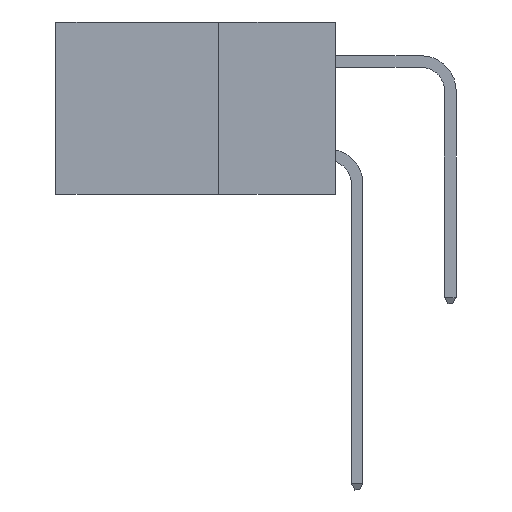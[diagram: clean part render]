
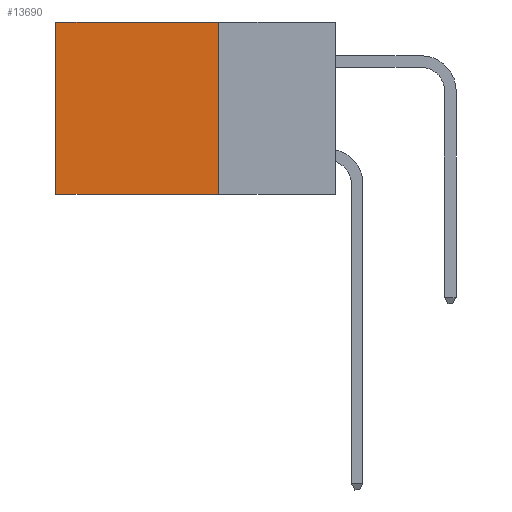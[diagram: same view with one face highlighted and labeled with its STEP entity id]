
A CAD part, left-side view. The second image highlights one B-rep face of the part: STEP entity #13690.
In plain terms, the highlighted planar face has unit normal (-1, 0, 0).
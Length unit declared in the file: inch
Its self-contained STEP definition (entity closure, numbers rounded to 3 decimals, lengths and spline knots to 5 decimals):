
#138 = DIRECTION ( 'NONE',  ( 0., 0., -1. ) ) ;
#770 = LINE ( 'NONE', #13454, #14005 ) ;
#819 = VERTEX_POINT ( 'NONE', #2191 ) ;
#1074 = PLANE ( 'NONE',  #18444 ) ;
#1243 = VECTOR ( 'NONE', #16279, 39.37008 ) ;
#2191 = CARTESIAN_POINT ( 'NONE',  ( 0.2875, 0.25, 0. ) ) ;
#2360 = DIRECTION ( 'NONE',  ( 0., 1., 0. ) ) ;
#2567 = EDGE_CURVE ( 'NONE', #5842, #14217, #11339, .T. ) ;
#2846 = DIRECTION ( 'NONE',  ( 1., 0., 0. ) ) ;
#4188 = EDGE_CURVE ( 'NONE', #8565, #14217, #14970, .T. ) ;
#4939 = ORIENTED_EDGE ( 'NONE', *, *, #13810, .F. ) ;
#5367 = CARTESIAN_POINT ( 'NONE',  ( 0.2875, 0.6, 0. ) ) ;
#5842 = VERTEX_POINT ( 'NONE', #19831 ) ;
#6802 = VECTOR ( 'NONE', #138, 39.37008 ) ;
#8030 = CARTESIAN_POINT ( 'NONE',  ( 0.2875, 0.25, 0. ) ) ;
#8565 = VERTEX_POINT ( 'NONE', #13923 ) ;
#10708 = ORIENTED_EDGE ( 'NONE', *, *, #4188, .F. ) ;
#11164 = CARTESIAN_POINT ( 'NONE',  ( 0.2875, 0.25, -0.37 ) ) ;
#11339 = LINE ( 'NONE', #5367, #6802 ) ;
#12298 = EDGE_CURVE ( 'NONE', #819, #5842, #13822, .T. ) ;
#12642 = EDGE_LOOP ( 'NONE', ( #20370, #10708, #4939, #18631 ) ) ;
#13294 = VECTOR ( 'NONE', #2360, 39.37008 ) ;
#13454 = CARTESIAN_POINT ( 'NONE',  ( 0.2875, 0.25, 0. ) ) ;
#13690 = ADVANCED_FACE ( 'NONE', ( #15603 ), #1074, .F. ) ;
#13810 = EDGE_CURVE ( 'NONE', #819, #8565, #770, .T. ) ;
#13822 = LINE ( 'NONE', #16030, #13294 ) ;
#13923 = CARTESIAN_POINT ( 'NONE',  ( 0.2875, 0.25, -0.37 ) ) ;
#14005 = VECTOR ( 'NONE', #20160, 39.37008 ) ;
#14217 = VERTEX_POINT ( 'NONE', #21177 ) ;
#14852 = DIRECTION ( 'NONE',  ( 0., 0., -1. ) ) ;
#14970 = LINE ( 'NONE', #11164, #1243 ) ;
#15603 = FACE_OUTER_BOUND ( 'NONE', #12642, .T. ) ;
#16030 = CARTESIAN_POINT ( 'NONE',  ( 0.2875, 0.25, 0. ) ) ;
#16279 = DIRECTION ( 'NONE',  ( 0., 1., 0. ) ) ;
#18444 = AXIS2_PLACEMENT_3D ( 'NONE', #8030, #2846, #14852 ) ;
#18631 = ORIENTED_EDGE ( 'NONE', *, *, #12298, .T. ) ;
#19831 = CARTESIAN_POINT ( 'NONE',  ( 0.2875, 0.6, 0. ) ) ;
#20160 = DIRECTION ( 'NONE',  ( 0., 0., -1. ) ) ;
#20370 = ORIENTED_EDGE ( 'NONE', *, *, #2567, .T. ) ;
#21177 = CARTESIAN_POINT ( 'NONE',  ( 0.2875, 0.6, -0.37 ) ) ;
